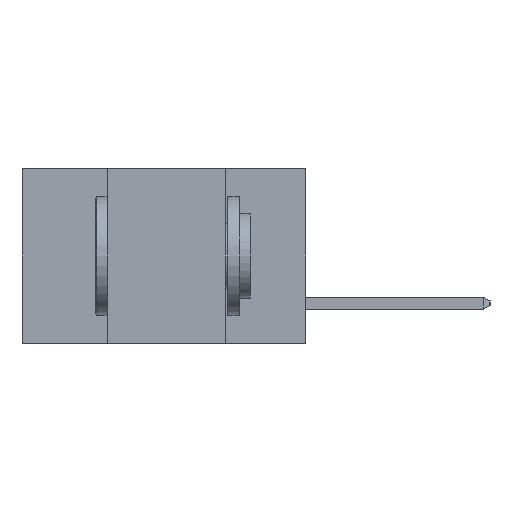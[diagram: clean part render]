
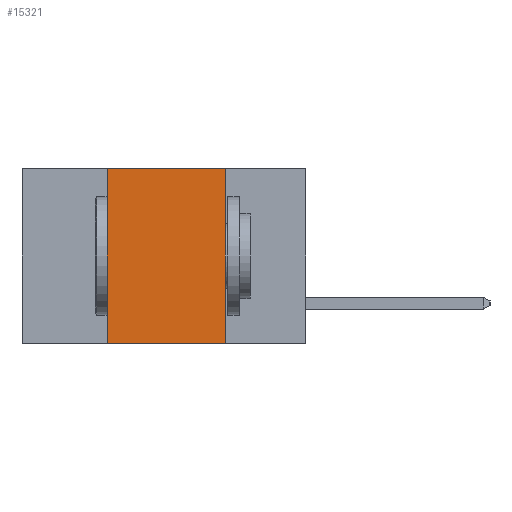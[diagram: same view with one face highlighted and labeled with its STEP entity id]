
A CAD part, left-side view. The second image highlights one B-rep face of the part: STEP entity #15321.
In plain terms, the highlighted planar face has unit normal (-1, 0, 0).
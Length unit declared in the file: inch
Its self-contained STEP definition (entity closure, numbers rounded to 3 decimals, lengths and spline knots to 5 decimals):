
#420 = CARTESIAN_POINT ( 'NONE',  ( 0., 0.6, -0.37 ) ) ;
#730 = FACE_OUTER_BOUND ( 'NONE', #7649, .T. ) ;
#1963 = EDGE_CURVE ( 'NONE', #2696, #2774, #4921, .T. ) ;
#2162 = LINE ( 'NONE', #19725, #9865 ) ;
#2696 = VERTEX_POINT ( 'NONE', #2975 ) ;
#2774 = VERTEX_POINT ( 'NONE', #3465 ) ;
#2975 = CARTESIAN_POINT ( 'NONE',  ( 0., 0.42, -0.37 ) ) ;
#3043 = DIRECTION ( 'NONE',  ( 0., 0., 1. ) ) ;
#3200 = VECTOR ( 'NONE', #3043, 39.37008 ) ;
#3465 = CARTESIAN_POINT ( 'NONE',  ( 0., 0.17, -0.37 ) ) ;
#4441 = EDGE_CURVE ( 'NONE', #2696, #15076, #8082, .T. ) ;
#4921 = LINE ( 'NONE', #420, #14634 ) ;
#5285 = DIRECTION ( 'NONE',  ( 0., 0., -1. ) ) ;
#5905 = CARTESIAN_POINT ( 'NONE',  ( 0., 0.6, 0. ) ) ;
#7649 = EDGE_LOOP ( 'NONE', ( #10130, #22604, #17978, #22037 ) ) ;
#7792 = DIRECTION ( 'NONE',  ( 0., -1., 0. ) ) ;
#8082 = LINE ( 'NONE', #13192, #3200 ) ;
#8126 = DIRECTION ( 'NONE',  ( 0., -1., 0. ) ) ;
#9118 = DIRECTION ( 'NONE',  ( 0., 0., -1. ) ) ;
#9404 = EDGE_CURVE ( 'NONE', #21605, #2774, #2162, .T. ) ;
#9634 = EDGE_CURVE ( 'NONE', #15076, #21605, #14365, .T. ) ;
#9865 = VECTOR ( 'NONE', #5285, 39.37008 ) ;
#10130 = ORIENTED_EDGE ( 'NONE', *, *, #9404, .F. ) ;
#10255 = CARTESIAN_POINT ( 'NONE',  ( 0., 0.42, 0. ) ) ;
#13192 = CARTESIAN_POINT ( 'NONE',  ( 0., 0.42, 0. ) ) ;
#14365 = LINE ( 'NONE', #5905, #23193 ) ;
#14634 = VECTOR ( 'NONE', #8126, 39.37008 ) ;
#15076 = VERTEX_POINT ( 'NONE', #10255 ) ;
#15321 = ADVANCED_FACE ( 'NONE', ( #730 ), #18072, .F. ) ;
#15744 = CARTESIAN_POINT ( 'NONE',  ( 0., 0.17, 0. ) ) ;
#16261 = CARTESIAN_POINT ( 'NONE',  ( 0., 0.6, 0. ) ) ;
#17978 = ORIENTED_EDGE ( 'NONE', *, *, #4441, .F. ) ;
#18072 = PLANE ( 'NONE',  #18741 ) ;
#18741 = AXIS2_PLACEMENT_3D ( 'NONE', #16261, #19819, #9118 ) ;
#19725 = CARTESIAN_POINT ( 'NONE',  ( 0., 0.17, 0. ) ) ;
#19819 = DIRECTION ( 'NONE',  ( 1., 0., 0. ) ) ;
#21605 = VERTEX_POINT ( 'NONE', #15744 ) ;
#22037 = ORIENTED_EDGE ( 'NONE', *, *, #1963, .T. ) ;
#22604 = ORIENTED_EDGE ( 'NONE', *, *, #9634, .F. ) ;
#23193 = VECTOR ( 'NONE', #7792, 39.37008 ) ;
